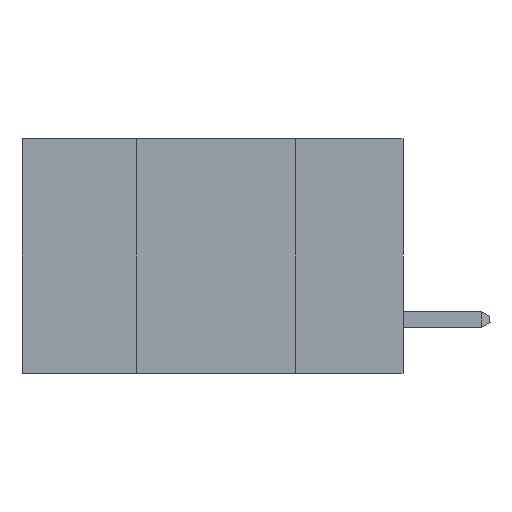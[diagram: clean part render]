
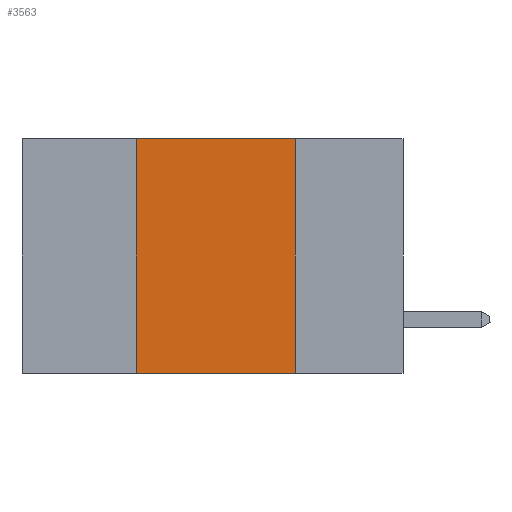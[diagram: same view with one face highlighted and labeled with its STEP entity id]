
A CAD part, left-side view. The second image highlights one B-rep face of the part: STEP entity #3563.
In plain terms, the highlighted planar face has unit normal (-1, 0, 0).
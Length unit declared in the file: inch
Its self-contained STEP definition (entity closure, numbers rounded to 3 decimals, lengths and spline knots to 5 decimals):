
#1379 = EDGE_CURVE ( 'NONE', #9043, #28602, #7426, .T. ) ;
#2118 = ORIENTED_EDGE ( 'NONE', *, *, #1379, .F. ) ;
#2853 = CARTESIAN_POINT ( 'NONE',  ( 0., 0.17, -0.37 ) ) ;
#3563 = ADVANCED_FACE ( 'NONE', ( #26414 ), #24694, .F. ) ;
#4169 = VERTEX_POINT ( 'NONE', #21923 ) ;
#5179 = CARTESIAN_POINT ( 'NONE',  ( 0., 0.42, -0.37 ) ) ;
#5208 = AXIS2_PLACEMENT_3D ( 'NONE', #42794, #6542, #28289 ) ;
#6188 = VERTEX_POINT ( 'NONE', #5179 ) ;
#6542 = DIRECTION ( 'NONE',  ( 1., 0., 0. ) ) ;
#7426 = LINE ( 'NONE', #20263, #23796 ) ;
#9043 = VERTEX_POINT ( 'NONE', #19739 ) ;
#10837 = EDGE_CURVE ( 'NONE', #6188, #4169, #29955, .T. ) ;
#14590 = LINE ( 'NONE', #22841, #43869 ) ;
#15275 = VECTOR ( 'NONE', #21055, 39.37008 ) ;
#16321 = DIRECTION ( 'NONE',  ( 0., -1., 0. ) ) ;
#17462 = VECTOR ( 'NONE', #16321, 39.37008 ) ;
#18537 = LINE ( 'NONE', #20276, #17462 ) ;
#18675 = EDGE_LOOP ( 'NONE', ( #2118, #30173, #24024, #36584 ) ) ;
#19739 = CARTESIAN_POINT ( 'NONE',  ( 0., 0.17, 0. ) ) ;
#20263 = CARTESIAN_POINT ( 'NONE',  ( 0., 0.17, 0. ) ) ;
#20276 = CARTESIAN_POINT ( 'NONE',  ( 0., 0.6, 0. ) ) ;
#21055 = DIRECTION ( 'NONE',  ( 0., 0., 1. ) ) ;
#21923 = CARTESIAN_POINT ( 'NONE',  ( 0., 0.42, 0. ) ) ;
#22841 = CARTESIAN_POINT ( 'NONE',  ( 0., 0.6, -0.37 ) ) ;
#23796 = VECTOR ( 'NONE', #38460, 39.37008 ) ;
#23953 = EDGE_CURVE ( 'NONE', #6188, #28602, #14590, .T. ) ;
#24024 = ORIENTED_EDGE ( 'NONE', *, *, #10837, .F. ) ;
#24694 = PLANE ( 'NONE',  #5208 ) ;
#26414 = FACE_OUTER_BOUND ( 'NONE', #18675, .T. ) ;
#28289 = DIRECTION ( 'NONE',  ( 0., 0., -1. ) ) ;
#28602 = VERTEX_POINT ( 'NONE', #2853 ) ;
#29955 = LINE ( 'NONE', #41756, #15275 ) ;
#30173 = ORIENTED_EDGE ( 'NONE', *, *, #38181, .F. ) ;
#34741 = DIRECTION ( 'NONE',  ( 0., -1., 0. ) ) ;
#36584 = ORIENTED_EDGE ( 'NONE', *, *, #23953, .T. ) ;
#38181 = EDGE_CURVE ( 'NONE', #4169, #9043, #18537, .T. ) ;
#38460 = DIRECTION ( 'NONE',  ( 0., 0., -1. ) ) ;
#41756 = CARTESIAN_POINT ( 'NONE',  ( 0., 0.42, 0. ) ) ;
#42794 = CARTESIAN_POINT ( 'NONE',  ( 0., 0.6, 0. ) ) ;
#43869 = VECTOR ( 'NONE', #34741, 39.37008 ) ;
